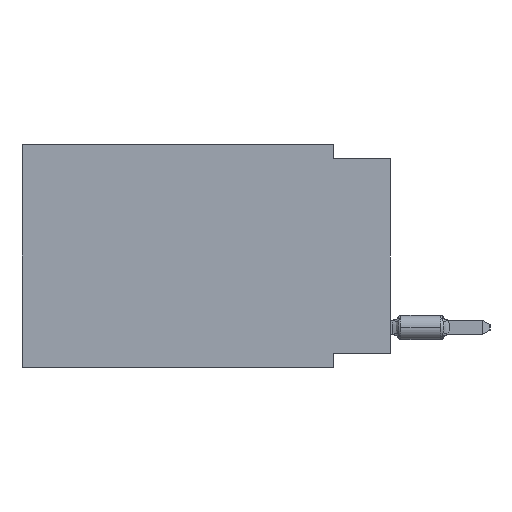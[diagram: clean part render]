
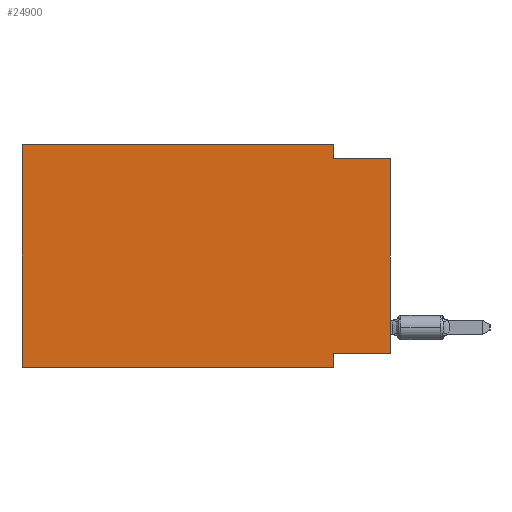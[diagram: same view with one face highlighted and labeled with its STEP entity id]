
A CAD part, left-side view. The second image highlights one B-rep face of the part: STEP entity #24900.
In plain terms, the highlighted planar face has unit normal (-1, 0, 0).
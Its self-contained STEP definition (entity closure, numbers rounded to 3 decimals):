
#511 = CARTESIAN_POINT ( 'NONE',  ( 0., 2.54, 0. ) ) ;
#2939 = VERTEX_POINT ( 'NONE', #46413 ) ;
#3585 = DIRECTION ( 'NONE',  ( 0., -1., 0. ) ) ;
#3706 = EDGE_CURVE ( 'NONE', #2939, #13531, #37077, .T. ) ;
#4028 = DIRECTION ( 'NONE',  ( 0., 0., -1. ) ) ;
#4242 = LINE ( 'NONE', #8293, #42599 ) ;
#5469 = CARTESIAN_POINT ( 'NONE',  ( 0., 16.383, -9.906 ) ) ;
#5657 = LINE ( 'NONE', #45118, #36348 ) ;
#6314 = CARTESIAN_POINT ( 'NONE',  ( 0., 0., -0.635 ) ) ;
#7544 = CARTESIAN_POINT ( 'NONE',  ( 0., 0., -9.271 ) ) ;
#7674 = VERTEX_POINT ( 'NONE', #36262 ) ;
#7843 = ORIENTED_EDGE ( 'NONE', *, *, #8059, .F. ) ;
#8059 = EDGE_CURVE ( 'NONE', #34753, #22752, #10723, .T. ) ;
#8288 = VERTEX_POINT ( 'NONE', #5469 ) ;
#8293 = CARTESIAN_POINT ( 'NONE',  ( 0., 0., -9.271 ) ) ;
#9429 = AXIS2_PLACEMENT_3D ( 'NONE', #29784, #31747, #39116 ) ;
#9887 = ORIENTED_EDGE ( 'NONE', *, *, #13459, .F. ) ;
#10078 = EDGE_CURVE ( 'NONE', #8288, #13531, #41365, .T. ) ;
#10113 = PLANE ( 'NONE',  #9429 ) ;
#10500 = EDGE_CURVE ( 'NONE', #25755, #2939, #4242, .T. ) ;
#10723 = LINE ( 'NONE', #32832, #31825 ) ;
#12650 = CARTESIAN_POINT ( 'NONE',  ( 0., 2.54, 0. ) ) ;
#12907 = ORIENTED_EDGE ( 'NONE', *, *, #3706, .F. ) ;
#13459 = EDGE_CURVE ( 'NONE', #22752, #38809, #45218, .T. ) ;
#13531 = VERTEX_POINT ( 'NONE', #20981 ) ;
#14319 = EDGE_CURVE ( 'NONE', #8288, #34753, #14516, .T. ) ;
#14516 = LINE ( 'NONE', #33304, #24046 ) ;
#15480 = DIRECTION ( 'NONE',  ( 0., -1., 0. ) ) ;
#16752 = VECTOR ( 'NONE', #15480, 1000. ) ;
#18604 = VECTOR ( 'NONE', #20272, 1000. ) ;
#20272 = DIRECTION ( 'NONE',  ( 0., 0., -1. ) ) ;
#20981 = CARTESIAN_POINT ( 'NONE',  ( 0., 2.54, -9.906 ) ) ;
#22427 = FACE_OUTER_BOUND ( 'NONE', #41187, .T. ) ;
#22752 = VERTEX_POINT ( 'NONE', #511 ) ;
#22864 = CARTESIAN_POINT ( 'NONE',  ( 0., 16.383, -9.906 ) ) ;
#23919 = LINE ( 'NONE', #6314, #39688 ) ;
#24046 = VECTOR ( 'NONE', #36142, 1000. ) ;
#24900 = ADVANCED_FACE ( 'NONE', ( #22427 ), #10113, .F. ) ;
#25755 = VERTEX_POINT ( 'NONE', #7544 ) ;
#29784 = CARTESIAN_POINT ( 'NONE',  ( 0., 16.383, 0. ) ) ;
#31111 = ORIENTED_EDGE ( 'NONE', *, *, #14319, .F. ) ;
#31747 = DIRECTION ( 'NONE',  ( 1., 0., 0. ) ) ;
#31825 = VECTOR ( 'NONE', #3585, 1000. ) ;
#32832 = CARTESIAN_POINT ( 'NONE',  ( 0., 16.383, 0. ) ) ;
#33304 = CARTESIAN_POINT ( 'NONE',  ( 0., 16.383, 0. ) ) ;
#33800 = ORIENTED_EDGE ( 'NONE', *, *, #45126, .T. ) ;
#33988 = CARTESIAN_POINT ( 'NONE',  ( 0., 2.54, -9.906 ) ) ;
#34753 = VERTEX_POINT ( 'NONE', #45601 ) ;
#36142 = DIRECTION ( 'NONE',  ( 0., 0., 1. ) ) ;
#36262 = CARTESIAN_POINT ( 'NONE',  ( 0., 0., -0.635 ) ) ;
#36348 = VECTOR ( 'NONE', #38684, 1000. ) ;
#37077 = LINE ( 'NONE', #33988, #45250 ) ;
#37738 = DIRECTION ( 'NONE',  ( 0., 1., 0. ) ) ;
#38684 = DIRECTION ( 'NONE',  ( 0., 0., 1. ) ) ;
#38809 = VERTEX_POINT ( 'NONE', #39667 ) ;
#39116 = DIRECTION ( 'NONE',  ( 0., 0., -1. ) ) ;
#39667 = CARTESIAN_POINT ( 'NONE',  ( 0., 2.54, -0.635 ) ) ;
#39688 = VECTOR ( 'NONE', #41956, 1000. ) ;
#41187 = EDGE_LOOP ( 'NONE', ( #33800, #46103, #9887, #7843, #31111, #41503, #12907, #42641 ) ) ;
#41365 = LINE ( 'NONE', #22864, #16752 ) ;
#41503 = ORIENTED_EDGE ( 'NONE', *, *, #10078, .T. ) ;
#41956 = DIRECTION ( 'NONE',  ( 0., -1., 0. ) ) ;
#42599 = VECTOR ( 'NONE', #37738, 1000. ) ;
#42641 = ORIENTED_EDGE ( 'NONE', *, *, #10500, .F. ) ;
#45118 = CARTESIAN_POINT ( 'NONE',  ( 0., 0., 0. ) ) ;
#45126 = EDGE_CURVE ( 'NONE', #25755, #7674, #5657, .T. ) ;
#45218 = LINE ( 'NONE', #12650, #18604 ) ;
#45250 = VECTOR ( 'NONE', #4028, 1000. ) ;
#45601 = CARTESIAN_POINT ( 'NONE',  ( 0., 16.383, 0. ) ) ;
#46103 = ORIENTED_EDGE ( 'NONE', *, *, #46680, .F. ) ;
#46413 = CARTESIAN_POINT ( 'NONE',  ( 0., 2.54, -9.271 ) ) ;
#46680 = EDGE_CURVE ( 'NONE', #38809, #7674, #23919, .T. ) ;
